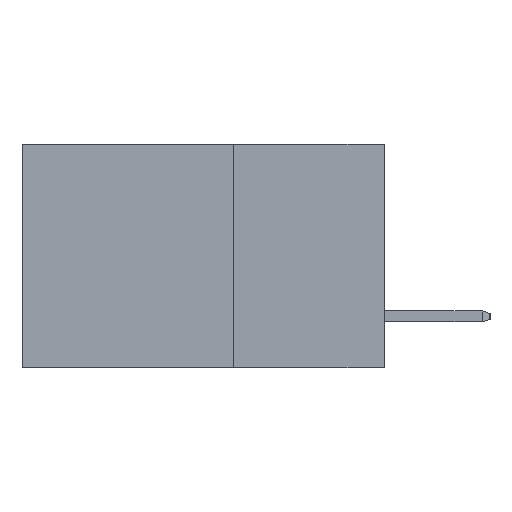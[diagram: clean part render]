
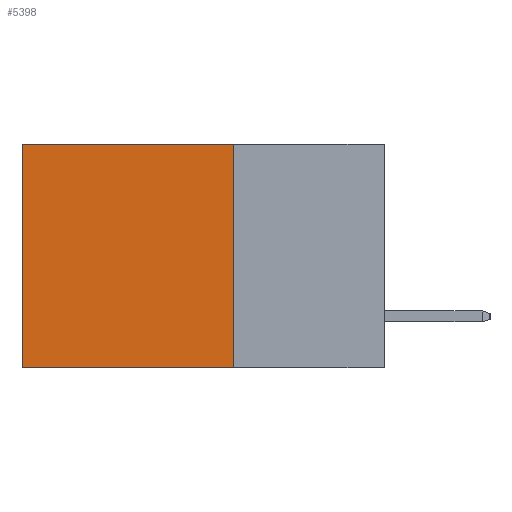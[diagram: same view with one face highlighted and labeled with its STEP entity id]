
A CAD part, left-side view. The second image highlights one B-rep face of the part: STEP entity #5398.
In plain terms, the highlighted planar face has unit normal (-1, 0, 0).
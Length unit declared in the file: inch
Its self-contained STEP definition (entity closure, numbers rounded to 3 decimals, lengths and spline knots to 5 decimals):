
#776 = ORIENTED_EDGE ( 'NONE', *, *, #13304, .T. ) ;
#886 = VERTEX_POINT ( 'NONE', #4673 ) ;
#934 = CARTESIAN_POINT ( 'NONE',  ( 0.2615, 0.25, -0.37 ) ) ;
#1401 = LINE ( 'NONE', #14135, #15469 ) ;
#1580 = VERTEX_POINT ( 'NONE', #934 ) ;
#1618 = AXIS2_PLACEMENT_3D ( 'NONE', #11732, #11557, #11545 ) ;
#2875 = LINE ( 'NONE', #17011, #17117 ) ;
#2935 = ORIENTED_EDGE ( 'NONE', *, *, #7719, .T. ) ;
#3053 = VERTEX_POINT ( 'NONE', #10190 ) ;
#4333 = ORIENTED_EDGE ( 'NONE', *, *, #14410, .F. ) ;
#4673 = CARTESIAN_POINT ( 'NONE',  ( 0.2615, 0.6, 0. ) ) ;
#5246 = CARTESIAN_POINT ( 'NONE',  ( 0.2615, 0.25, 0. ) ) ;
#5398 = ADVANCED_FACE ( 'NONE', ( #7290 ), #11745, .F. ) ;
#6385 = CARTESIAN_POINT ( 'NONE',  ( 0.2615, 0.25, -0.37 ) ) ;
#7290 = FACE_OUTER_BOUND ( 'NONE', #7589, .T. ) ;
#7589 = EDGE_LOOP ( 'NONE', ( #776, #14172, #4333, #2935 ) ) ;
#7719 = EDGE_CURVE ( 'NONE', #9405, #886, #1401, .T. ) ;
#9186 = DIRECTION ( 'NONE',  ( 0., 0., -1. ) ) ;
#9405 = VERTEX_POINT ( 'NONE', #5246 ) ;
#10094 = CARTESIAN_POINT ( 'NONE',  ( 0.2615, 0.25, -0.37 ) ) ;
#10190 = CARTESIAN_POINT ( 'NONE',  ( 0.2615, 0.6, -0.37 ) ) ;
#10279 = DIRECTION ( 'NONE',  ( 0., 1., 0. ) ) ;
#10306 = VECTOR ( 'NONE', #15650, 39.37008 ) ;
#10515 = EDGE_CURVE ( 'NONE', #1580, #3053, #14026, .T. ) ;
#11545 = DIRECTION ( 'NONE',  ( 0., 0., -1. ) ) ;
#11557 = DIRECTION ( 'NONE',  ( 1., 0., 0. ) ) ;
#11732 = CARTESIAN_POINT ( 'NONE',  ( 0.2615, 0.25, -0.37 ) ) ;
#11745 = PLANE ( 'NONE',  #1618 ) ;
#13304 = EDGE_CURVE ( 'NONE', #886, #3053, #2875, .T. ) ;
#13968 = DIRECTION ( 'NONE',  ( 0., 1., 0. ) ) ;
#14026 = LINE ( 'NONE', #10094, #17409 ) ;
#14135 = CARTESIAN_POINT ( 'NONE',  ( 0.2615, 0.25, 0. ) ) ;
#14172 = ORIENTED_EDGE ( 'NONE', *, *, #10515, .F. ) ;
#14410 = EDGE_CURVE ( 'NONE', #9405, #1580, #17210, .T. ) ;
#15469 = VECTOR ( 'NONE', #13968, 39.37008 ) ;
#15650 = DIRECTION ( 'NONE',  ( 0., 0., -1. ) ) ;
#17011 = CARTESIAN_POINT ( 'NONE',  ( 0.2615, 0.6, -0.37 ) ) ;
#17117 = VECTOR ( 'NONE', #9186, 39.37008 ) ;
#17210 = LINE ( 'NONE', #6385, #10306 ) ;
#17409 = VECTOR ( 'NONE', #10279, 39.37008 ) ;
